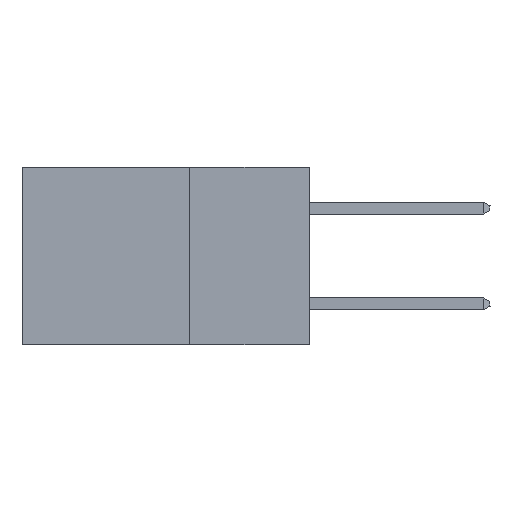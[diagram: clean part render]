
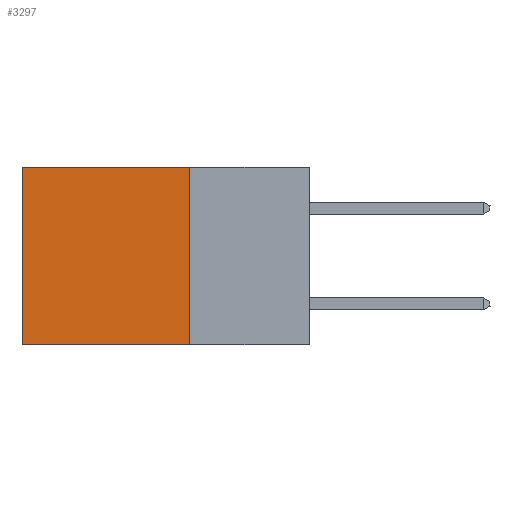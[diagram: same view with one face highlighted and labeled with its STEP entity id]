
A CAD part, left-side view. The second image highlights one B-rep face of the part: STEP entity #3297.
In plain terms, the highlighted planar face has unit normal (-1, 0, 0).
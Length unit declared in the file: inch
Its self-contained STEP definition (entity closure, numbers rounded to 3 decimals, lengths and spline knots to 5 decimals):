
#348 = VECTOR ( 'NONE', #16328, 39.37008 ) ;
#428 = ORIENTED_EDGE ( 'NONE', *, *, #19366, .F. ) ;
#1455 = VERTEX_POINT ( 'NONE', #14175 ) ;
#2380 = ORIENTED_EDGE ( 'NONE', *, *, #13342, .F. ) ;
#3106 = ORIENTED_EDGE ( 'NONE', *, *, #8886, .T. ) ;
#3161 = VECTOR ( 'NONE', #10672, 39.37008 ) ;
#3297 = ADVANCED_FACE ( 'NONE', ( #4670 ), #4766, .F. ) ;
#3975 = LINE ( 'NONE', #9328, #348 ) ;
#4495 = CARTESIAN_POINT ( 'NONE',  ( 0.2875, 0.6, -0.37 ) ) ;
#4670 = FACE_OUTER_BOUND ( 'NONE', #20790, .T. ) ;
#4766 = PLANE ( 'NONE',  #15610 ) ;
#5392 = ORIENTED_EDGE ( 'NONE', *, *, #17666, .T. ) ;
#5755 = LINE ( 'NONE', #18579, #18291 ) ;
#8740 = LINE ( 'NONE', #10749, #3161 ) ;
#8857 = VERTEX_POINT ( 'NONE', #19789 ) ;
#8886 = EDGE_CURVE ( 'NONE', #1455, #19617, #3975, .T. ) ;
#8907 = VECTOR ( 'NONE', #17242, 39.37008 ) ;
#9138 = CARTESIAN_POINT ( 'NONE',  ( 0.2875, 0.6, 0. ) ) ;
#9328 = CARTESIAN_POINT ( 'NONE',  ( 0.2875, 0.25, 0. ) ) ;
#10325 = CARTESIAN_POINT ( 'NONE',  ( 0.2875, 0.25, 0. ) ) ;
#10672 = DIRECTION ( 'NONE',  ( 0., 1., 0. ) ) ;
#10749 = CARTESIAN_POINT ( 'NONE',  ( 0.2875, 0.25, -0.37 ) ) ;
#11603 = VERTEX_POINT ( 'NONE', #4495 ) ;
#13342 = EDGE_CURVE ( 'NONE', #8857, #11603, #8740, .T. ) ;
#14175 = CARTESIAN_POINT ( 'NONE',  ( 0.2875, 0.25, 0. ) ) ;
#15610 = AXIS2_PLACEMENT_3D ( 'NONE', #18637, #20444, #17061 ) ;
#16328 = DIRECTION ( 'NONE',  ( 0., 1., 0. ) ) ;
#17061 = DIRECTION ( 'NONE',  ( 0., 0., -1. ) ) ;
#17242 = DIRECTION ( 'NONE',  ( 0., 0., -1. ) ) ;
#17666 = EDGE_CURVE ( 'NONE', #19617, #11603, #5755, .T. ) ;
#18291 = VECTOR ( 'NONE', #18655, 39.37008 ) ;
#18579 = CARTESIAN_POINT ( 'NONE',  ( 0.2875, 0.6, 0. ) ) ;
#18637 = CARTESIAN_POINT ( 'NONE',  ( 0.2875, 0.25, 0. ) ) ;
#18655 = DIRECTION ( 'NONE',  ( 0., 0., -1. ) ) ;
#19366 = EDGE_CURVE ( 'NONE', #1455, #8857, #22350, .T. ) ;
#19617 = VERTEX_POINT ( 'NONE', #9138 ) ;
#19789 = CARTESIAN_POINT ( 'NONE',  ( 0.2875, 0.25, -0.37 ) ) ;
#20444 = DIRECTION ( 'NONE',  ( 1., 0., 0. ) ) ;
#20790 = EDGE_LOOP ( 'NONE', ( #5392, #2380, #428, #3106 ) ) ;
#22350 = LINE ( 'NONE', #10325, #8907 ) ;
